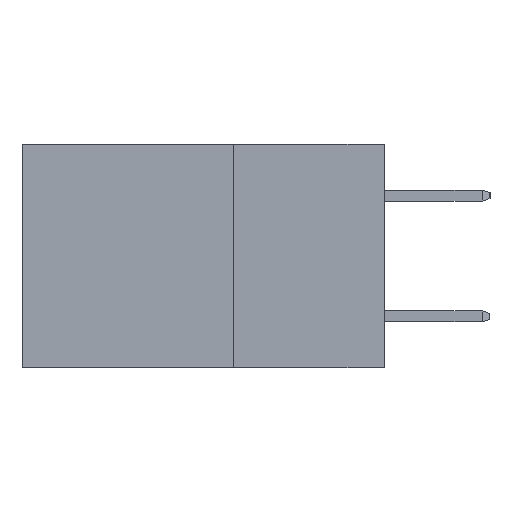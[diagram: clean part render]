
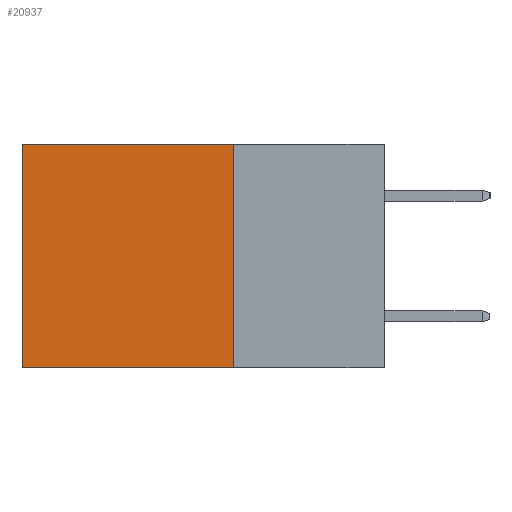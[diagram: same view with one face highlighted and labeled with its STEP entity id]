
A CAD part, left-side view. The second image highlights one B-rep face of the part: STEP entity #20937.
In plain terms, the highlighted planar face has unit normal (-1, 0, 0).
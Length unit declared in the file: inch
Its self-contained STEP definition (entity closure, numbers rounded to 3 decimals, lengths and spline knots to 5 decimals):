
#2247 = DIRECTION ( 'NONE',  ( 0., 0., -1. ) ) ;
#2743 = VERTEX_POINT ( 'NONE', #8061 ) ;
#3647 = LINE ( 'NONE', #11246, #19909 ) ;
#4457 = EDGE_CURVE ( 'NONE', #13552, #2743, #3647, .T. ) ;
#5372 = LINE ( 'NONE', #16434, #17804 ) ;
#6448 = ORIENTED_EDGE ( 'NONE', *, *, #4457, .T. ) ;
#6749 = ORIENTED_EDGE ( 'NONE', *, *, #13611, .F. ) ;
#7134 = VERTEX_POINT ( 'NONE', #12895 ) ;
#7240 = CARTESIAN_POINT ( 'NONE',  ( 0.298, 0.25, 0. ) ) ;
#8061 = CARTESIAN_POINT ( 'NONE',  ( 0.298, 0.6, -0.37 ) ) ;
#8342 = VECTOR ( 'NONE', #18570, 39.37008 ) ;
#9601 = FACE_OUTER_BOUND ( 'NONE', #19457, .T. ) ;
#10451 = CARTESIAN_POINT ( 'NONE',  ( 0.298, 0.25, 0. ) ) ;
#10462 = VECTOR ( 'NONE', #16716, 39.37008 ) ;
#11246 = CARTESIAN_POINT ( 'NONE',  ( 0.298, 0.6, 0. ) ) ;
#11355 = DIRECTION ( 'NONE',  ( 0., 0., -1. ) ) ;
#12083 = DIRECTION ( 'NONE',  ( 1., 0., 0. ) ) ;
#12115 = VERTEX_POINT ( 'NONE', #17841 ) ;
#12736 = ORIENTED_EDGE ( 'NONE', *, *, #14999, .T. ) ;
#12895 = CARTESIAN_POINT ( 'NONE',  ( 0.298, 0.25, 0. ) ) ;
#13552 = VERTEX_POINT ( 'NONE', #18207 ) ;
#13611 = EDGE_CURVE ( 'NONE', #12115, #2743, #14732, .T. ) ;
#14147 = ORIENTED_EDGE ( 'NONE', *, *, #18734, .F. ) ;
#14732 = LINE ( 'NONE', #15085, #10462 ) ;
#14999 = EDGE_CURVE ( 'NONE', #7134, #13552, #16419, .T. ) ;
#15085 = CARTESIAN_POINT ( 'NONE',  ( 0.298, 0.25, -0.37 ) ) ;
#16419 = LINE ( 'NONE', #7240, #8342 ) ;
#16434 = CARTESIAN_POINT ( 'NONE',  ( 0.298, 0.25, 0. ) ) ;
#16612 = AXIS2_PLACEMENT_3D ( 'NONE', #10451, #12083, #2247 ) ;
#16716 = DIRECTION ( 'NONE',  ( 0., 1., 0. ) ) ;
#17804 = VECTOR ( 'NONE', #18070, 39.37008 ) ;
#17841 = CARTESIAN_POINT ( 'NONE',  ( 0.298, 0.25, -0.37 ) ) ;
#18070 = DIRECTION ( 'NONE',  ( 0., 0., -1. ) ) ;
#18207 = CARTESIAN_POINT ( 'NONE',  ( 0.298, 0.6, 0. ) ) ;
#18570 = DIRECTION ( 'NONE',  ( 0., 1., 0. ) ) ;
#18734 = EDGE_CURVE ( 'NONE', #7134, #12115, #5372, .T. ) ;
#19457 = EDGE_LOOP ( 'NONE', ( #6448, #6749, #14147, #12736 ) ) ;
#19909 = VECTOR ( 'NONE', #11355, 39.37008 ) ;
#20090 = PLANE ( 'NONE',  #16612 ) ;
#20937 = ADVANCED_FACE ( 'NONE', ( #9601 ), #20090, .F. ) ;
